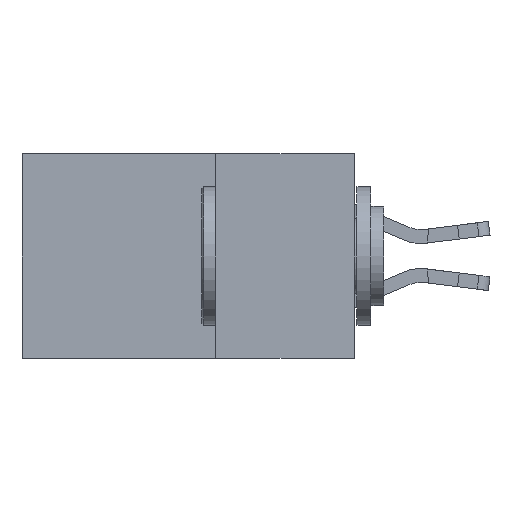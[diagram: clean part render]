
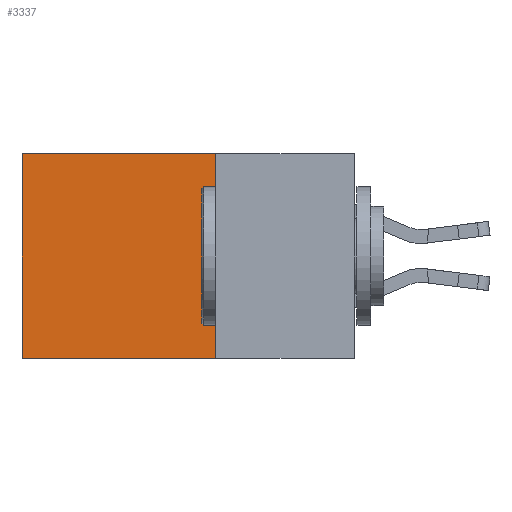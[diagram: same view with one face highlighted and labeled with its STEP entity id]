
A CAD part, left-side view. The second image highlights one B-rep face of the part: STEP entity #3337.
In plain terms, the highlighted planar face has unit normal (-1, 0, 0).
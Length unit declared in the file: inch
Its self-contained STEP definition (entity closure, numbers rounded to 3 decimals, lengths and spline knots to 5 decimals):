
#1675 = CARTESIAN_POINT ( 'NONE',  ( 0.2615, 0.6, -0.37 ) ) ;
#2182 = CARTESIAN_POINT ( 'NONE',  ( 0.2615, 0.25, -0.37 ) ) ;
#2534 = VECTOR ( 'NONE', #4294, 39.37008 ) ;
#3337 = ADVANCED_FACE ( 'NONE', ( #4755 ), #3365, .F. ) ;
#3365 = PLANE ( 'NONE',  #6377 ) ;
#3456 = EDGE_LOOP ( 'NONE', ( #10690, #3564, #8211, #9749 ) ) ;
#3564 = ORIENTED_EDGE ( 'NONE', *, *, #4091, .F. ) ;
#4091 = EDGE_CURVE ( 'NONE', #12604, #12632, #7440, .T. ) ;
#4294 = DIRECTION ( 'NONE',  ( 0., 1., 0. ) ) ;
#4541 = VECTOR ( 'NONE', #8061, 39.37008 ) ;
#4755 = FACE_OUTER_BOUND ( 'NONE', #3456, .T. ) ;
#4869 = VERTEX_POINT ( 'NONE', #13144 ) ;
#5594 = LINE ( 'NONE', #14365, #2534 ) ;
#6133 = CARTESIAN_POINT ( 'NONE',  ( 0.2615, 0.25, -0.37 ) ) ;
#6377 = AXIS2_PLACEMENT_3D ( 'NONE', #8349, #15977, #12122 ) ;
#7268 = DIRECTION ( 'NONE',  ( 0., 0., -1. ) ) ;
#7440 = LINE ( 'NONE', #6133, #10807 ) ;
#8061 = DIRECTION ( 'NONE',  ( 0., 0., -1. ) ) ;
#8211 = ORIENTED_EDGE ( 'NONE', *, *, #8633, .F. ) ;
#8349 = CARTESIAN_POINT ( 'NONE',  ( 0.2615, 0.25, -0.37 ) ) ;
#8633 = EDGE_CURVE ( 'NONE', #4869, #12604, #8652, .T. ) ;
#8652 = LINE ( 'NONE', #2182, #14973 ) ;
#9749 = ORIENTED_EDGE ( 'NONE', *, *, #15326, .T. ) ;
#10140 = EDGE_CURVE ( 'NONE', #10205, #12632, #12000, .T. ) ;
#10205 = VERTEX_POINT ( 'NONE', #10694 ) ;
#10402 = CARTESIAN_POINT ( 'NONE',  ( 0.2615, 0.25, -0.37 ) ) ;
#10690 = ORIENTED_EDGE ( 'NONE', *, *, #10140, .T. ) ;
#10694 = CARTESIAN_POINT ( 'NONE',  ( 0.2615, 0.6, 0. ) ) ;
#10807 = VECTOR ( 'NONE', #14902, 39.37008 ) ;
#12000 = LINE ( 'NONE', #1675, #4541 ) ;
#12122 = DIRECTION ( 'NONE',  ( 0., 0., -1. ) ) ;
#12604 = VERTEX_POINT ( 'NONE', #10402 ) ;
#12632 = VERTEX_POINT ( 'NONE', #12953 ) ;
#12953 = CARTESIAN_POINT ( 'NONE',  ( 0.2615, 0.6, -0.37 ) ) ;
#13144 = CARTESIAN_POINT ( 'NONE',  ( 0.2615, 0.25, 0. ) ) ;
#14365 = CARTESIAN_POINT ( 'NONE',  ( 0.2615, 0.25, 0. ) ) ;
#14902 = DIRECTION ( 'NONE',  ( 0., 1., 0. ) ) ;
#14973 = VECTOR ( 'NONE', #7268, 39.37008 ) ;
#15326 = EDGE_CURVE ( 'NONE', #4869, #10205, #5594, .T. ) ;
#15977 = DIRECTION ( 'NONE',  ( 1., 0., 0. ) ) ;
